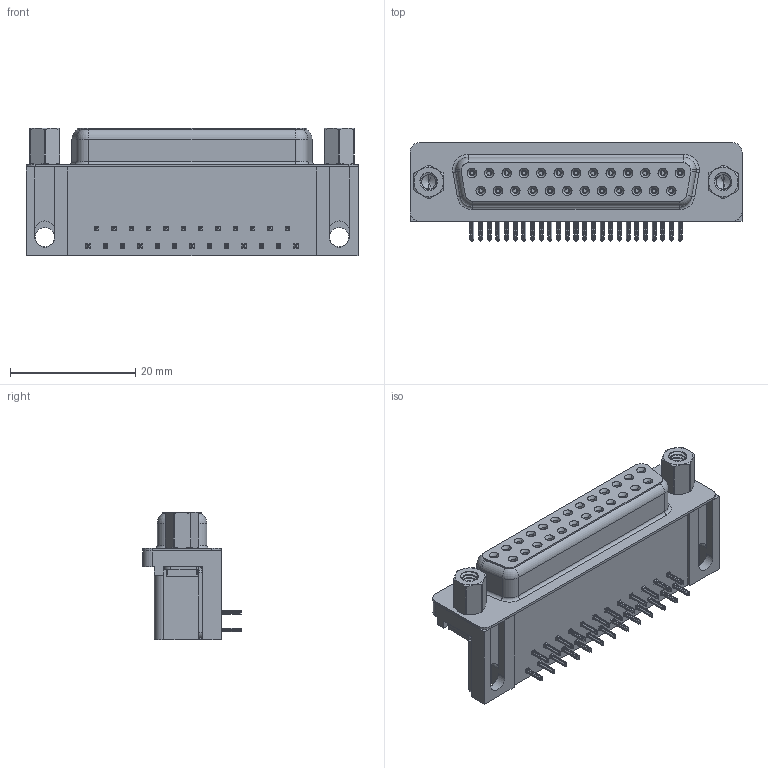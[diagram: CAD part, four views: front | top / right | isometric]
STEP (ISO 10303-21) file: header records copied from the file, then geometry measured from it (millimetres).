
FILE_DESCRIPTION (( 'STEP AP203' ), '1' );
FILE_NAME ('630-025-340-513.STEP', '2021-09-22T14:04:25', ( '' ), ( '' ), 'SwSTEP 2.0', 'SolidWorks 2020', '' );
FILE_SCHEMA (( 'CONFIG_CONTROL_DESIGN' ));
Length unit declared in the file: millimetre
Products named in the file (8): 630 Housing_25 Socket; 630 Shell_25 Socket; 630 Thru Hole Board Mount; 630 4-40 Hex Standoff 5; 630 Contact Top; 630-025-340-513; 630 4-40 Threaded Rivet; 630 Contact Bottom
Assembly tree (33 placements, depth 2):
  630-025-340-513
    630 Housing_25 Socket
    630 Shell_25 Socket
    630 Contact Bottom  x12
    630 Contact Top  x13
    630 Thru Hole Board Mount  x2
    630 4-40 Threaded Rivet  x2
    630 4-40 Hex Standoff 5  x2
Bounding box: 53.04 x 15.73 x 20.4 mm (x, y, z)
Volume: 8800.8 mm3; surface area: 10556.6 mm2
Topology: 33 solids, 33 shells, 3976 faces, 10452 edges, 6562 vertices
Faces by surface type: plane 1744, cylinder 992, bspline 870, cone 332, torus 38
Entity records: 35663 total; most frequent: CARTESIAN_POINT 12937, ORIENTED_EDGE 4556, DIRECTION 4103, EDGE_CURVE 2278, VERTEX_POINT 1457, VECTOR 1417, LINE 1417, AXIS2_PLACEMENT_3D 1343
